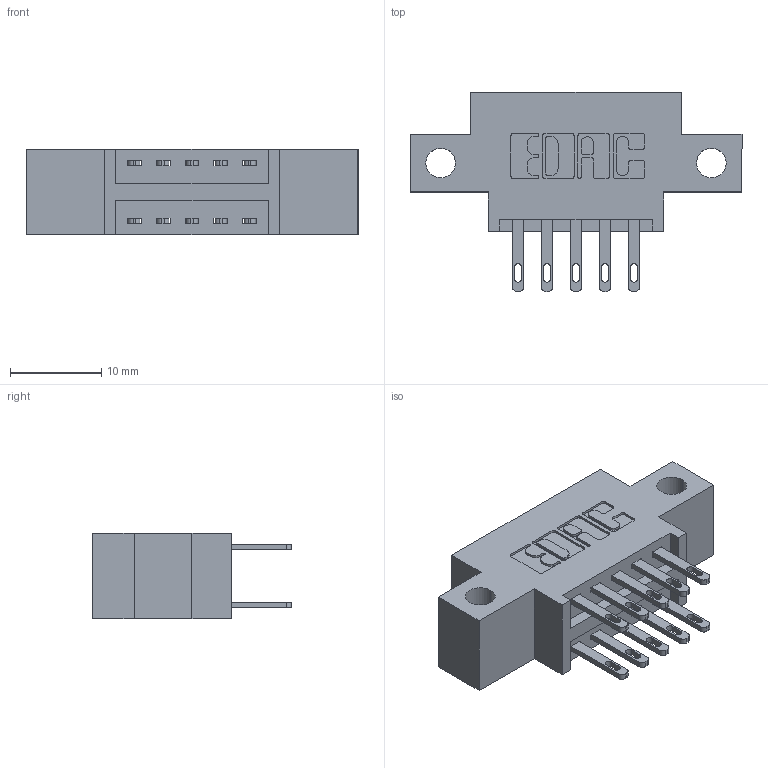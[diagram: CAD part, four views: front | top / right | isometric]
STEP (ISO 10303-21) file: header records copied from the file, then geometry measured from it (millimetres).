
FILE_DESCRIPTION (( 'STEP AP203' ), '1' );
FILE_NAME ('346-010-500-812.STEP', '2018-08-17T06:18:48', ( '' ), ( '' ), 'SwSTEP 2.0', 'SolidWorks 2016', '' );
FILE_SCHEMA (( 'CONFIG_CONTROL_DESIGN' ));
Length unit declared in the file: inch
Products named in the file (3): 345-292-001_345-293-100; 346-010-500-812; 346 Part_0.170 Offset - Side Mount
Assembly tree (11 placements, depth 2):
  346-010-500-812
    346 Part_0.170 Offset - Side Mount
    345-292-001_345-293-100  x10
Bounding box: 36.45 x 21.84 x 9.4 mm (x, y, z)
Volume: 3055.5 mm3; surface area: 3765.3 mm2
Topology: 11 solids, 11 shells, 606 faces, 1811 edges, 1206 vertices
Faces by surface type: plane 370, cylinder 236
Entity records: 8309 total; most frequent: CARTESIAN_POINT 1420, ORIENTED_EDGE 1354, DIRECTION 1305, EDGE_CURVE 677, VECTOR 521, LINE 521, VERTEX_POINT 450, AXIS2_PLACEMENT_3D 392
